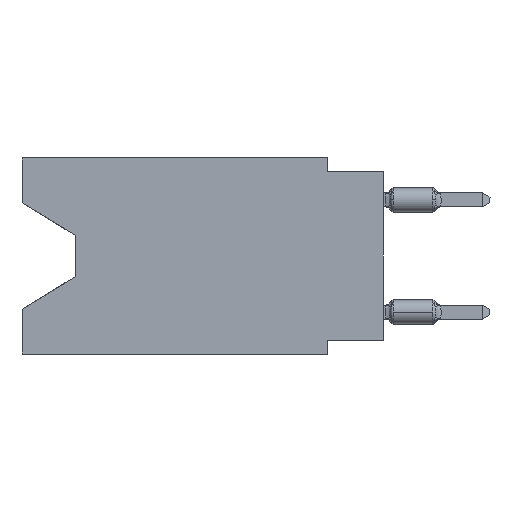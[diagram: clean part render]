
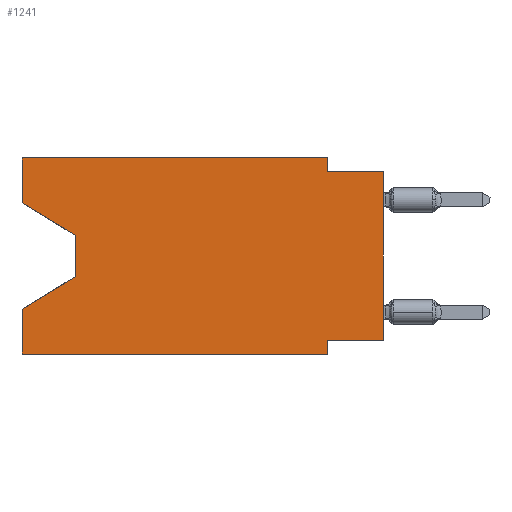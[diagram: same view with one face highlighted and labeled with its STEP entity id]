
A CAD part, left-side view. The second image highlights one B-rep face of the part: STEP entity #1241.
In plain terms, the highlighted planar face has unit normal (-1, 0, 0).
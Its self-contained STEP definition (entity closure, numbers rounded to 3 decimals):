
#69 = EDGE_CURVE ( 'NONE', #4110, #14441, #3845, .T. ) ;
#234 = AXIS2_PLACEMENT_3D ( 'NONE', #12179, #14610, #3031 ) ;
#245 = LINE ( 'NONE', #8397, #8072 ) ;
#263 = EDGE_CURVE ( 'NONE', #2296, #4110, #11619, .T. ) ;
#1028 = CARTESIAN_POINT ( 'NONE',  ( 0., 16.383, -8.89 ) ) ;
#1127 = ORIENTED_EDGE ( 'NONE', *, *, #7864, .F. ) ;
#1150 = VERTEX_POINT ( 'NONE', #13689 ) ;
#1234 = CARTESIAN_POINT ( 'NONE',  ( 0., 16.383, 0. ) ) ;
#1241 = ADVANCED_FACE ( 'NONE', ( #4183 ), #14471, .F. ) ;
#1344 = VECTOR ( 'NONE', #6659, 1000. ) ;
#1403 = CARTESIAN_POINT ( 'NONE',  ( 0., 16.383, 0. ) ) ;
#1731 = VERTEX_POINT ( 'NONE', #1234 ) ;
#2083 = CARTESIAN_POINT ( 'NONE',  ( 0., 2.54, 0. ) ) ;
#2296 = VERTEX_POINT ( 'NONE', #8369 ) ;
#2387 = CARTESIAN_POINT ( 'NONE',  ( 0., 16.383, 0. ) ) ;
#2422 = ORIENTED_EDGE ( 'NONE', *, *, #8645, .T. ) ;
#2460 = LINE ( 'NONE', #5979, #3444 ) ;
#2618 = LINE ( 'NONE', #1403, #4510 ) ;
#2965 = VERTEX_POINT ( 'NONE', #6429 ) ;
#3031 = DIRECTION ( 'NONE',  ( 0., 0., -1. ) ) ;
#3304 = DIRECTION ( 'NONE',  ( 0., 0., -1. ) ) ;
#3444 = VECTOR ( 'NONE', #4684, 1000. ) ;
#3770 = VECTOR ( 'NONE', #7037, 1000. ) ;
#3840 = EDGE_CURVE ( 'NONE', #9117, #4558, #10185, .T. ) ;
#3845 = LINE ( 'NONE', #7367, #8341 ) ;
#4110 = VERTEX_POINT ( 'NONE', #9577 ) ;
#4183 = FACE_OUTER_BOUND ( 'NONE', #7594, .T. ) ;
#4205 = CARTESIAN_POINT ( 'NONE',  ( 0., 2.54, -8.89 ) ) ;
#4311 = VERTEX_POINT ( 'NONE', #14963 ) ;
#4351 = VERTEX_POINT ( 'NONE', #1028 ) ;
#4384 = ORIENTED_EDGE ( 'NONE', *, *, #4586, .T. ) ;
#4388 = DIRECTION ( 'NONE',  ( 0., 0., -1. ) ) ;
#4437 = EDGE_CURVE ( 'NONE', #1731, #2296, #2618, .T. ) ;
#4510 = VECTOR ( 'NONE', #10700, 1000. ) ;
#4558 = VERTEX_POINT ( 'NONE', #9561 ) ;
#4586 = EDGE_CURVE ( 'NONE', #4558, #4311, #11847, .T. ) ;
#4663 = VECTOR ( 'NONE', #4670, 1000. ) ;
#4670 = DIRECTION ( 'NONE',  ( 0., 0., -1. ) ) ;
#4684 = DIRECTION ( 'NONE',  ( 0., -0.855, -0.519 ) ) ;
#4732 = EDGE_CURVE ( 'NONE', #8157, #1150, #14635, .T. ) ;
#5298 = CARTESIAN_POINT ( 'NONE',  ( 0., 0., -8.255 ) ) ;
#5544 = CARTESIAN_POINT ( 'NONE',  ( 0., 13.97, -3.505 ) ) ;
#5874 = VECTOR ( 'NONE', #13970, 1000. ) ;
#5979 = CARTESIAN_POINT ( 'NONE',  ( 0., 16.383, -2.038 ) ) ;
#6023 = CARTESIAN_POINT ( 'NONE',  ( 0., 16.383, 0. ) ) ;
#6052 = CARTESIAN_POINT ( 'NONE',  ( 0., 13.97, -5.385 ) ) ;
#6185 = ORIENTED_EDGE ( 'NONE', *, *, #263, .F. ) ;
#6429 = CARTESIAN_POINT ( 'NONE',  ( 0., 16.383, -2.038 ) ) ;
#6659 = DIRECTION ( 'NONE',  ( 0., -1., 0. ) ) ;
#6761 = VERTEX_POINT ( 'NONE', #5298 ) ;
#7002 = CARTESIAN_POINT ( 'NONE',  ( 0., 0., -0.635 ) ) ;
#7037 = DIRECTION ( 'NONE',  ( 0., 0., 1. ) ) ;
#7169 = ORIENTED_EDGE ( 'NONE', *, *, #14842, .F. ) ;
#7312 = LINE ( 'NONE', #6023, #9841 ) ;
#7367 = CARTESIAN_POINT ( 'NONE',  ( 0., 0., -0.635 ) ) ;
#7594 = EDGE_LOOP ( 'NONE', ( #14599, #10155, #4384, #1127, #8912, #9129, #9875, #2422, #11928, #6185, #12853, #7169 ) ) ;
#7864 = EDGE_CURVE ( 'NONE', #4351, #4311, #7312, .T. ) ;
#8072 = VECTOR ( 'NONE', #8696, 1000. ) ;
#8157 = VERTEX_POINT ( 'NONE', #13845 ) ;
#8341 = VECTOR ( 'NONE', #12007, 1000. ) ;
#8369 = CARTESIAN_POINT ( 'NONE',  ( 0., 2.54, 0. ) ) ;
#8379 = DIRECTION ( 'NONE',  ( 0., 0., 1. ) ) ;
#8397 = CARTESIAN_POINT ( 'NONE',  ( 0., 0., 0. ) ) ;
#8620 = EDGE_CURVE ( 'NONE', #6761, #8157, #12901, .T. ) ;
#8645 = EDGE_CURVE ( 'NONE', #6761, #14441, #245, .T. ) ;
#8696 = DIRECTION ( 'NONE',  ( 0., 0., 1. ) ) ;
#8702 = VECTOR ( 'NONE', #3304, 1000. ) ;
#8912 = ORIENTED_EDGE ( 'NONE', *, *, #14597, .T. ) ;
#9117 = VERTEX_POINT ( 'NONE', #5544 ) ;
#9129 = ORIENTED_EDGE ( 'NONE', *, *, #4732, .F. ) ;
#9330 = CARTESIAN_POINT ( 'NONE',  ( 0., 0., -8.255 ) ) ;
#9561 = CARTESIAN_POINT ( 'NONE',  ( 0., 13.97, -5.385 ) ) ;
#9577 = CARTESIAN_POINT ( 'NONE',  ( 0., 2.54, -0.635 ) ) ;
#9841 = VECTOR ( 'NONE', #8379, 1000. ) ;
#9875 = ORIENTED_EDGE ( 'NONE', *, *, #8620, .F. ) ;
#10155 = ORIENTED_EDGE ( 'NONE', *, *, #3840, .T. ) ;
#10185 = LINE ( 'NONE', #14818, #14475 ) ;
#10700 = DIRECTION ( 'NONE',  ( 0., -1., 0. ) ) ;
#10779 = DIRECTION ( 'NONE',  ( 0., 0.855, -0.519 ) ) ;
#11376 = LINE ( 'NONE', #13736, #1344 ) ;
#11619 = LINE ( 'NONE', #2083, #8702 ) ;
#11634 = EDGE_CURVE ( 'NONE', #2965, #9117, #2460, .T. ) ;
#11847 = LINE ( 'NONE', #6052, #12918 ) ;
#11928 = ORIENTED_EDGE ( 'NONE', *, *, #69, .F. ) ;
#12007 = DIRECTION ( 'NONE',  ( 0., -1., 0. ) ) ;
#12179 = CARTESIAN_POINT ( 'NONE',  ( 0., 16.383, 0. ) ) ;
#12834 = LINE ( 'NONE', #2387, #3770 ) ;
#12853 = ORIENTED_EDGE ( 'NONE', *, *, #4437, .F. ) ;
#12901 = LINE ( 'NONE', #9330, #5874 ) ;
#12918 = VECTOR ( 'NONE', #10779, 1000. ) ;
#13689 = CARTESIAN_POINT ( 'NONE',  ( 0., 2.54, -8.89 ) ) ;
#13736 = CARTESIAN_POINT ( 'NONE',  ( 0., 16.383, -8.89 ) ) ;
#13845 = CARTESIAN_POINT ( 'NONE',  ( 0., 2.54, -8.255 ) ) ;
#13970 = DIRECTION ( 'NONE',  ( 0., 1., 0. ) ) ;
#14441 = VERTEX_POINT ( 'NONE', #7002 ) ;
#14471 = PLANE ( 'NONE',  #234 ) ;
#14475 = VECTOR ( 'NONE', #4388, 1000. ) ;
#14597 = EDGE_CURVE ( 'NONE', #4351, #1150, #11376, .T. ) ;
#14599 = ORIENTED_EDGE ( 'NONE', *, *, #11634, .T. ) ;
#14610 = DIRECTION ( 'NONE',  ( 1., 0., 0. ) ) ;
#14635 = LINE ( 'NONE', #4205, #4663 ) ;
#14818 = CARTESIAN_POINT ( 'NONE',  ( 0., 13.97, -3.505 ) ) ;
#14842 = EDGE_CURVE ( 'NONE', #2965, #1731, #12834, .T. ) ;
#14963 = CARTESIAN_POINT ( 'NONE',  ( 0., 16.383, -6.852 ) ) ;
